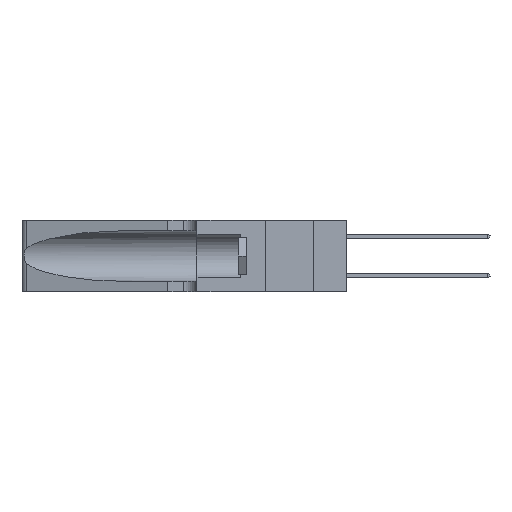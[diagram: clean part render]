
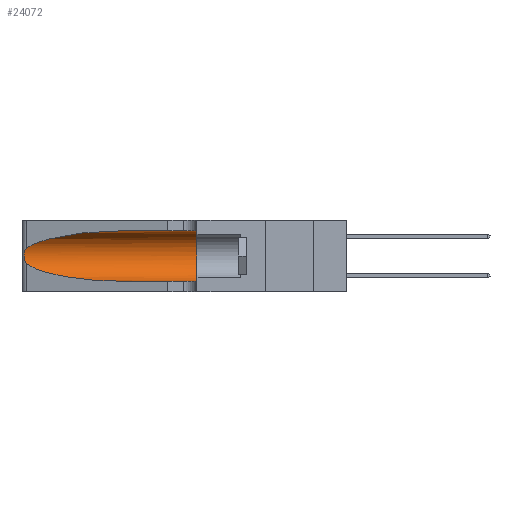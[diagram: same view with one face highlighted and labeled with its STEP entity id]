
A CAD part, left-side view. The second image highlights one B-rep face of the part: STEP entity #24072.
In plain terms, the highlighted cylindrical face has radius 3.308 mm (diameter 6.617 mm), a partial arc.
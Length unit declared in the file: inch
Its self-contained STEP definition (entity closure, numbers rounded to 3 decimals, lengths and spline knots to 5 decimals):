
#27 = CARTESIAN_POINT ( 'NONE',  ( 0.25487, 1.22718, 0.22369 ) ) ;
#280 = CARTESIAN_POINT ( 'NONE',  ( 0.1305, 0.35, 0.31525 ) ) ;
#362 = CARTESIAN_POINT ( 'NONE',  ( 0.1305, 0.72297, 0.31525 ) ) ;
#409 = CARTESIAN_POINT ( 'NONE',  ( 0.25856, 1.23593, 0.16098 ) ) ;
#1705 = VERTEX_POINT ( 'NONE', #35397 ) ;
#1961 = DIRECTION ( 'NONE',  ( 0., -1., 0. ) ) ;
#2036 = DIRECTION ( 'NONE',  ( 0., -1., 0. ) ) ;
#2691 = CARTESIAN_POINT ( 'NONE',  ( 0.2373, 1.15595, 0.28018 ) ) ;
#3221 = CARTESIAN_POINT ( 'NONE',  ( 0.25487, 1.22718, 0.22369 ) ) ;
#3341 = CARTESIAN_POINT ( 'NONE',  ( 0.25639, 1.23186, 0.15144 ) ) ;
#3509 = DIRECTION ( 'NONE',  ( 0., 0., 1. ) ) ;
#3762 = VERTEX_POINT ( 'NONE', #6241 ) ;
#4005 = VECTOR ( 'NONE', #15448, 39.37008 ) ;
#4275 = ORIENTED_EDGE ( 'NONE', *, *, #27947, .T. ) ;
#5011 = VERTEX_POINT ( 'NONE', #27571 ) ;
#5277 = FACE_OUTER_BOUND ( 'NONE', #30081, .T. ) ;
#5321 = ORIENTED_EDGE ( 'NONE', *, *, #23962, .T. ) ;
#5367 = DIRECTION ( 'NONE',  ( 0., 1., 0. ) ) ;
#5964 = CARTESIAN_POINT ( 'NONE',  ( 0.25639, 1.23184, 0.21858 ) ) ;
#6023 = VECTOR ( 'NONE', #1961, 39.37008 ) ;
#6241 = CARTESIAN_POINT ( 'NONE',  ( 0.1305, 0.72297, 0.05475 ) ) ;
#6325 = CARTESIAN_POINT ( 'NONE',  ( 0.26075, 1.23896, 0.19203 ) ) ;
#6739 = CARTESIAN_POINT ( 'NONE',  ( 0.1305, 0.35, 0.185 ) ) ;
#7651 = CARTESIAN_POINT ( 'NONE',  ( 0.1305, 1.61858, 0.31525 ) ) ;
#8799 = CARTESIAN_POINT ( 'NONE',  ( 0.25555, 1.22993, 0.14849 ) ) ;
#8943 = AXIS2_PLACEMENT_3D ( 'NONE', #6739, #5367, #3509 ) ;
#9563 = ORIENTED_EDGE ( 'NONE', *, *, #17856, .F. ) ;
#10222 = CARTESIAN_POINT ( 'NONE',  ( 0.1305, 0.72297, 0.31525 ) ) ;
#11482 = CARTESIAN_POINT ( 'NONE',  ( 0.25787, 1.23484, 0.2124 ) ) ;
#11600 = CARTESIAN_POINT ( 'NONE',  ( 0.26075, 1.23896, 0.178 ) ) ;
#13626 = EDGE_CURVE ( 'NONE', #1705, #3762, #28610, .T. ) ;
#13961 = CIRCLE ( 'NONE', #8943, 0.13025 ) ;
#14481 = ORIENTED_EDGE ( 'NONE', *, *, #25308, .F. ) ;
#15335 = VERTEX_POINT ( 'NONE', #34090 ) ;
#15448 = DIRECTION ( 'NONE',  ( 0., -1., 0. ) ) ;
#16480 = CARTESIAN_POINT ( 'NONE',  ( 0.1305, 1.61858, 0.185 ) ) ;
#17159 = CARTESIAN_POINT ( 'NONE',  ( 0.25854, 1.2359, 0.20912 ) ) ;
#17788 = LINE ( 'NONE', #7651, #6023 ) ;
#17856 = EDGE_CURVE ( 'NONE', #24817, #5011, #13961, .T. ) ;
#18728 = CYLINDRICAL_SURFACE ( 'NONE', #18825, 0.13025 ) ;
#18757 = CARTESIAN_POINT ( 'NONE',  ( 0.2373, 1.15595, 0.08982 ) ) ;
#18825 = AXIS2_PLACEMENT_3D ( 'NONE', #16480, #2036, #32578 ) ;
#19690 = CARTESIAN_POINT ( 'NONE',  ( 0.25789, 1.23486, 0.15765 ) ) ;
#20169 = CARTESIAN_POINT ( 'NONE',  ( 0.26018, 1.23835, 0.19895 ) ) ;
#21528 =( BOUNDED_CURVE ( )  B_SPLINE_CURVE ( 3, ( #362, #33589, #2691, #27 ),
 .UNSPECIFIED., .F., .T. ) 
 B_SPLINE_CURVE_WITH_KNOTS ( ( 4, 4 ),
 ( 1.5708, 2.84003 ),
 .UNSPECIFIED. ) 
 CURVE ( )  GEOMETRIC_REPRESENTATION_ITEM ( )  RATIONAL_B_SPLINE_CURVE ( ( 1., 0.87, 0.87, 1. ) ) 
 REPRESENTATION_ITEM ( '' )  );
#21572 = VERTEX_POINT ( 'NONE', #10222 ) ;
#22831 = CARTESIAN_POINT ( 'NONE',  ( 0.26017, 1.23833, 0.17102 ) ) ;
#23860 = ORIENTED_EDGE ( 'NONE', *, *, #13626, .T. ) ;
#23962 = EDGE_CURVE ( 'NONE', #3762, #5011, #31361, .T. ) ;
#24072 = ADVANCED_FACE ( 'NONE', ( #5277 ), #18728, .F. ) ;
#24313 = CARTESIAN_POINT ( 'NONE',  ( 0.18966, 0.96281, 0.05475 ) ) ;
#24817 = VERTEX_POINT ( 'NONE', #280 ) ;
#25308 = EDGE_CURVE ( 'NONE', #21572, #24817, #17788, .T. ) ;
#27220 = CARTESIAN_POINT ( 'NONE',  ( 0.25487, 1.22718, 0.14631 ) ) ;
#27571 = CARTESIAN_POINT ( 'NONE',  ( 0.1305, 0.35, 0.05475 ) ) ;
#27947 = EDGE_CURVE ( 'NONE', #15335, #1705, #29750, .T. ) ;
#28284 = CARTESIAN_POINT ( 'NONE',  ( 0.25555, 1.22994, 0.2215 ) ) ;
#28610 =( BOUNDED_CURVE ( )  B_SPLINE_CURVE ( 3, ( #27220, #18757, #24313, #29784 ),
 .UNSPECIFIED., .F., .F. ) 
 B_SPLINE_CURVE_WITH_KNOTS ( ( 4, 4 ),
 ( 3.44316, 4.71239 ),
 .UNSPECIFIED. ) 
 CURVE ( )  GEOMETRIC_REPRESENTATION_ITEM ( )  RATIONAL_B_SPLINE_CURVE ( ( 1., 0.87, 0.87, 1. ) ) 
 REPRESENTATION_ITEM ( '' )  );
#29201 = CARTESIAN_POINT ( 'NONE',  ( 0.1305, 1.61858, 0.05475 ) ) ;
#29750 = B_SPLINE_CURVE_WITH_KNOTS ( 'NONE', 3,
 ( #3221, #28284, #5964, #11482, #17159, #20169, #6325, #11600, #22831, #409, #19690, #3341, #8799, #33522 ),
 .UNSPECIFIED., .F., .F.,
 ( 4, 2, 2, 2, 2, 2, 4 ),
 ( 0., 0.00027, 0.00053, 0.00107, 0.0016, 0.00187, 0.00214 ),
 .UNSPECIFIED. ) ;
#29768 = ORIENTED_EDGE ( 'NONE', *, *, #35022, .T. ) ;
#29784 = CARTESIAN_POINT ( 'NONE',  ( 0.1305, 0.72297, 0.05475 ) ) ;
#30081 = EDGE_LOOP ( 'NONE', ( #29768, #4275, #23860, #5321, #9563, #14481 ) ) ;
#31361 = LINE ( 'NONE', #29201, #4005 ) ;
#32578 = DIRECTION ( 'NONE',  ( 0., 0., -1. ) ) ;
#33522 = CARTESIAN_POINT ( 'NONE',  ( 0.25487, 1.22718, 0.14631 ) ) ;
#33589 = CARTESIAN_POINT ( 'NONE',  ( 0.18966, 0.96281, 0.31525 ) ) ;
#34090 = CARTESIAN_POINT ( 'NONE',  ( 0.25487, 1.22718, 0.22369 ) ) ;
#35022 = EDGE_CURVE ( 'NONE', #21572, #15335, #21528, .T. ) ;
#35397 = CARTESIAN_POINT ( 'NONE',  ( 0.25487, 1.22718, 0.14631 ) ) ;
